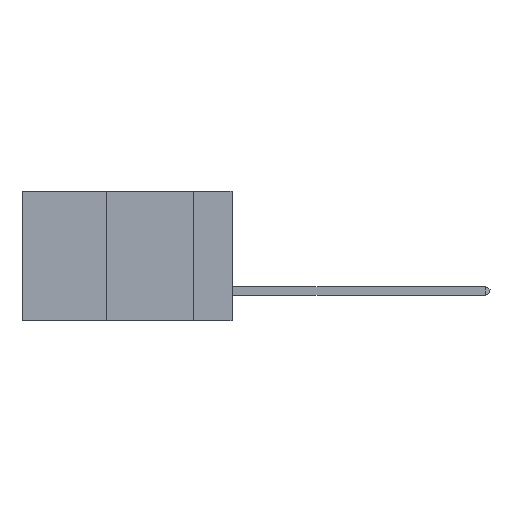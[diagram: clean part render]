
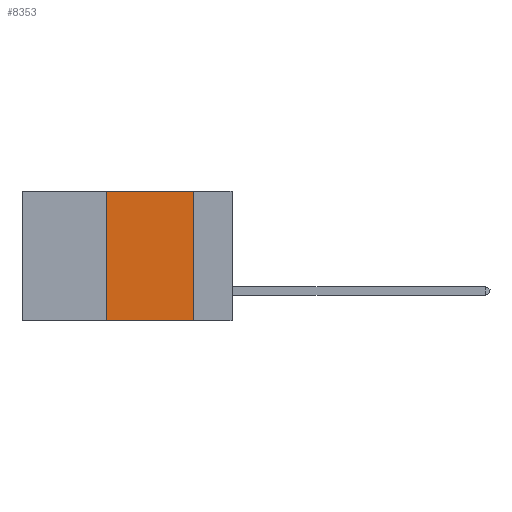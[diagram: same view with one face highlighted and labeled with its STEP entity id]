
A CAD part, left-side view. The second image highlights one B-rep face of the part: STEP entity #8353.
In plain terms, the highlighted planar face has unit normal (-1, 0, 0).
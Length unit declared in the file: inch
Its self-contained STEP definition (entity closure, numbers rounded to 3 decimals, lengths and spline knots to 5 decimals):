
#1215 = AXIS2_PLACEMENT_3D ( 'NONE', #5757, #9000, #2605 ) ;
#1392 = EDGE_CURVE ( 'NONE', #13097, #6270, #6532, .T. ) ;
#1623 = VERTEX_POINT ( 'NONE', #12470 ) ;
#1770 = VECTOR ( 'NONE', #4881, 39.37008 ) ;
#2122 = ORIENTED_EDGE ( 'NONE', *, *, #9026, .T. ) ;
#2411 = ORIENTED_EDGE ( 'NONE', *, *, #1392, .F. ) ;
#2605 = DIRECTION ( 'NONE',  ( 0., 0., -1. ) ) ;
#3118 = VERTEX_POINT ( 'NONE', #9801 ) ;
#3673 = VECTOR ( 'NONE', #12382, 39.37008 ) ;
#3704 = CARTESIAN_POINT ( 'NONE',  ( 0., 0.6, -0.37 ) ) ;
#4060 = ORIENTED_EDGE ( 'NONE', *, *, #5782, .F. ) ;
#4238 = ORIENTED_EDGE ( 'NONE', *, *, #13589, .F. ) ;
#4654 = LINE ( 'NONE', #3704, #1770 ) ;
#4881 = DIRECTION ( 'NONE',  ( 0., -1., 0. ) ) ;
#5757 = CARTESIAN_POINT ( 'NONE',  ( 0., 0.6, 0. ) ) ;
#5782 = EDGE_CURVE ( 'NONE', #1623, #3118, #8523, .T. ) ;
#6270 = VERTEX_POINT ( 'NONE', #12881 ) ;
#6323 = LINE ( 'NONE', #12939, #11974 ) ;
#6532 = LINE ( 'NONE', #10057, #3673 ) ;
#6957 = EDGE_LOOP ( 'NONE', ( #4060, #4238, #2411, #2122 ) ) ;
#7375 = VECTOR ( 'NONE', #7493, 39.37008 ) ;
#7493 = DIRECTION ( 'NONE',  ( 0., 0., -1. ) ) ;
#7792 = CARTESIAN_POINT ( 'NONE',  ( 0., 0.36, -0.37 ) ) ;
#8353 = ADVANCED_FACE ( 'NONE', ( #10638 ), #12220, .F. ) ;
#8523 = LINE ( 'NONE', #12721, #7375 ) ;
#9000 = DIRECTION ( 'NONE',  ( 1., 0., 0. ) ) ;
#9026 = EDGE_CURVE ( 'NONE', #13097, #3118, #4654, .T. ) ;
#9801 = CARTESIAN_POINT ( 'NONE',  ( 0., 0.11, -0.37 ) ) ;
#10057 = CARTESIAN_POINT ( 'NONE',  ( 0., 0.36, 0. ) ) ;
#10638 = FACE_OUTER_BOUND ( 'NONE', #6957, .T. ) ;
#11818 = DIRECTION ( 'NONE',  ( 0., -1., 0. ) ) ;
#11974 = VECTOR ( 'NONE', #11818, 39.37008 ) ;
#12220 = PLANE ( 'NONE',  #1215 ) ;
#12382 = DIRECTION ( 'NONE',  ( 0., 0., 1. ) ) ;
#12470 = CARTESIAN_POINT ( 'NONE',  ( 0., 0.11, 0. ) ) ;
#12721 = CARTESIAN_POINT ( 'NONE',  ( 0., 0.11, 0. ) ) ;
#12881 = CARTESIAN_POINT ( 'NONE',  ( 0., 0.36, 0. ) ) ;
#12939 = CARTESIAN_POINT ( 'NONE',  ( 0., 0.6, 0. ) ) ;
#13097 = VERTEX_POINT ( 'NONE', #7792 ) ;
#13589 = EDGE_CURVE ( 'NONE', #6270, #1623, #6323, .T. ) ;
